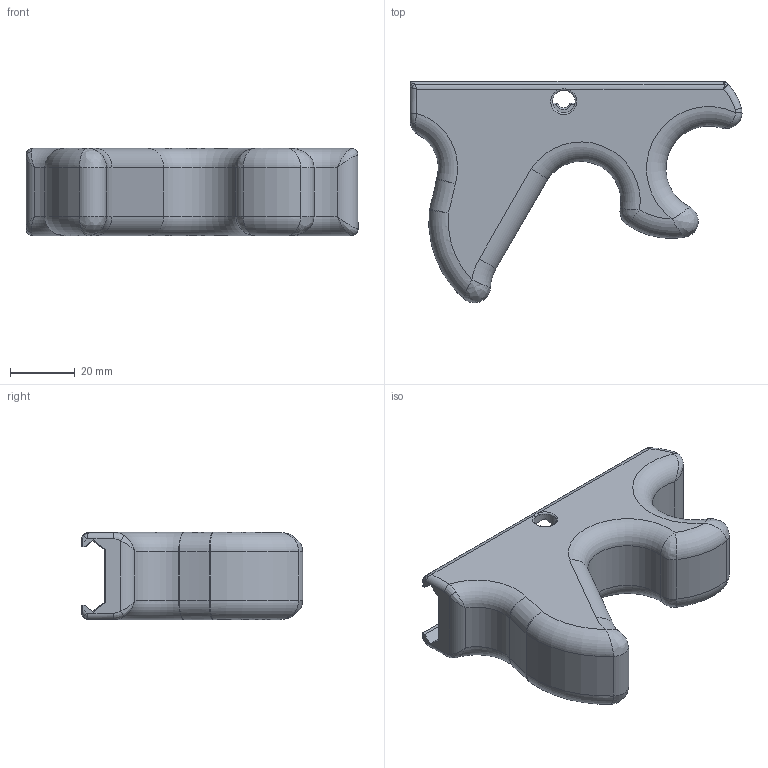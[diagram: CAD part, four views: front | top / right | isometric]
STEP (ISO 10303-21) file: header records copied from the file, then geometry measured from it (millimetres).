
FILE_DESCRIPTION(/* description */ ('STEP AP242','CAx-IF Rec.Pracs.---Representation and Presentation of Product Manufacturing Information (PMI)---4.0---2014-10-13','CAx-IF Rec.Pracs.---3D Tessellated Geometry---0.4---2014-09-14','2;1'),/* implementation_level */ '2;1');
FILE_NAME(/* name */ '632c3f6c42732454060c3a66',/* time_stamp */ '2022-09-22T10:56:45+00:00',/* author */ (''),/* organization */ (''),/* preprocessor_version */ 'ST-DEVELOPER v18.102',/* originating_system */ ' ',/* authorisation */ ' ');
FILE_SCHEMA (('AP242_MANAGED_MODEL_BASED_3D_ENGINEERING_MIM_LF { 1 0 10303 442 1 1 4 }'));
Length unit declared in the file: metre
Products named in the file (1): Part 1
Bounding box: 102.75 x 68.53 x 27 mm (x, y, z)
Volume: 83885.4 mm3; surface area: 17173.9 mm2
Topology: 1 solids, 1 shells, 140 faces, 363 edges, 200 vertices
Faces by surface type: bspline 44, cylinder 41, plane 31, torus 21, sphere 3
Full cylindrical faces by diameter (mm): 7 x1
Entity records: 4842 total; most frequent: CARTESIAN_POINT 1779, ORIENTED_EDGE 678, DIRECTION 602, EDGE_CURVE 339, AXIS2_PLACEMENT_3D 239, VERTEX_POINT 198, EDGE_LOOP 141, FACE_BOUND 141
